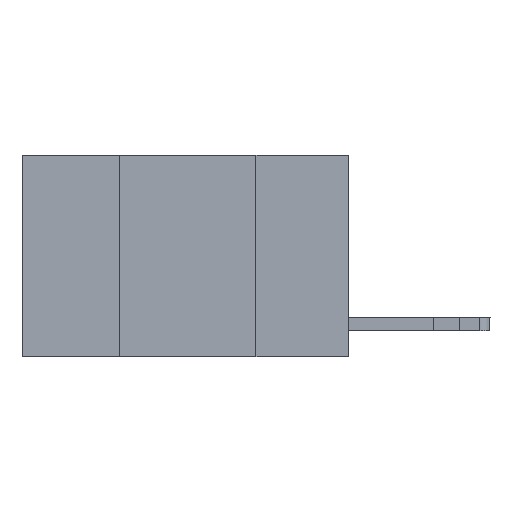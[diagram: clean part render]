
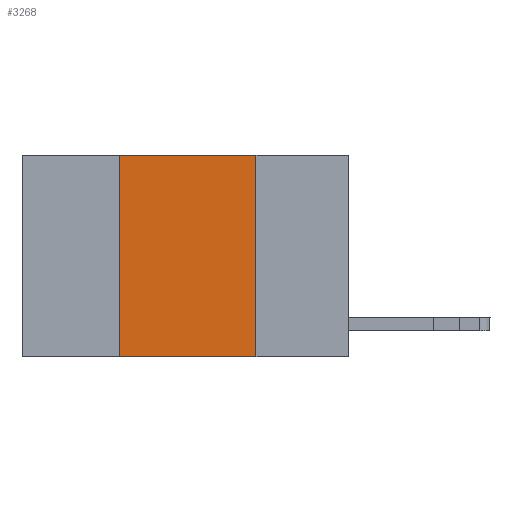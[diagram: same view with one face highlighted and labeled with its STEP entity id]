
A CAD part, left-side view. The second image highlights one B-rep face of the part: STEP entity #3268.
In plain terms, the highlighted planar face has unit normal (-1, 0, 0).
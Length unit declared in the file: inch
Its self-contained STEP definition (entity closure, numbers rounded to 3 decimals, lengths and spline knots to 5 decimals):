
#578 = CARTESIAN_POINT ( 'NONE',  ( 0., 0.17, -0.37 ) ) ;
#594 = VERTEX_POINT ( 'NONE', #4495 ) ;
#1509 = CARTESIAN_POINT ( 'NONE',  ( 0., 0.17, 0. ) ) ;
#1961 = DIRECTION ( 'NONE',  ( 1., 0., 0. ) ) ;
#2389 = VERTEX_POINT ( 'NONE', #578 ) ;
#2548 = LINE ( 'NONE', #1509, #4572 ) ;
#3052 = DIRECTION ( 'NONE',  ( 0., 0., -1. ) ) ;
#3268 = ADVANCED_FACE ( 'NONE', ( #13177 ), #10371, .F. ) ;
#3316 = VERTEX_POINT ( 'NONE', #5961 ) ;
#4274 = CARTESIAN_POINT ( 'NONE',  ( 0., 0.6, -0.37 ) ) ;
#4415 = EDGE_LOOP ( 'NONE', ( #5103, #5250, #9996, #11718 ) ) ;
#4495 = CARTESIAN_POINT ( 'NONE',  ( 0., 0.42, -0.37 ) ) ;
#4572 = VECTOR ( 'NONE', #12928, 39.37008 ) ;
#5103 = ORIENTED_EDGE ( 'NONE', *, *, #5426, .F. ) ;
#5250 = ORIENTED_EDGE ( 'NONE', *, *, #8561, .F. ) ;
#5426 = EDGE_CURVE ( 'NONE', #11020, #2389, #2548, .T. ) ;
#5708 = VECTOR ( 'NONE', #5855, 39.37008 ) ;
#5855 = DIRECTION ( 'NONE',  ( 0., 0., 1. ) ) ;
#5961 = CARTESIAN_POINT ( 'NONE',  ( 0., 0.42, 0. ) ) ;
#5977 = CARTESIAN_POINT ( 'NONE',  ( 0., 0.17, 0. ) ) ;
#6027 = CARTESIAN_POINT ( 'NONE',  ( 0., 0.6, 0. ) ) ;
#6548 = VECTOR ( 'NONE', #9359, 39.37008 ) ;
#6941 = CARTESIAN_POINT ( 'NONE',  ( 0., 0.42, 0. ) ) ;
#7397 = VECTOR ( 'NONE', #11466, 39.37008 ) ;
#8561 = EDGE_CURVE ( 'NONE', #3316, #11020, #10048, .T. ) ;
#9093 = EDGE_CURVE ( 'NONE', #594, #2389, #12473, .T. ) ;
#9359 = DIRECTION ( 'NONE',  ( 0., -1., 0. ) ) ;
#9996 = ORIENTED_EDGE ( 'NONE', *, *, #10580, .F. ) ;
#10048 = LINE ( 'NONE', #6027, #7397 ) ;
#10371 = PLANE ( 'NONE',  #12001 ) ;
#10580 = EDGE_CURVE ( 'NONE', #594, #3316, #11971, .T. ) ;
#11020 = VERTEX_POINT ( 'NONE', #5977 ) ;
#11466 = DIRECTION ( 'NONE',  ( 0., -1., 0. ) ) ;
#11718 = ORIENTED_EDGE ( 'NONE', *, *, #9093, .T. ) ;
#11971 = LINE ( 'NONE', #6941, #5708 ) ;
#12001 = AXIS2_PLACEMENT_3D ( 'NONE', #12290, #1961, #3052 ) ;
#12290 = CARTESIAN_POINT ( 'NONE',  ( 0., 0.6, 0. ) ) ;
#12473 = LINE ( 'NONE', #4274, #6548 ) ;
#12928 = DIRECTION ( 'NONE',  ( 0., 0., -1. ) ) ;
#13177 = FACE_OUTER_BOUND ( 'NONE', #4415, .T. ) ;
